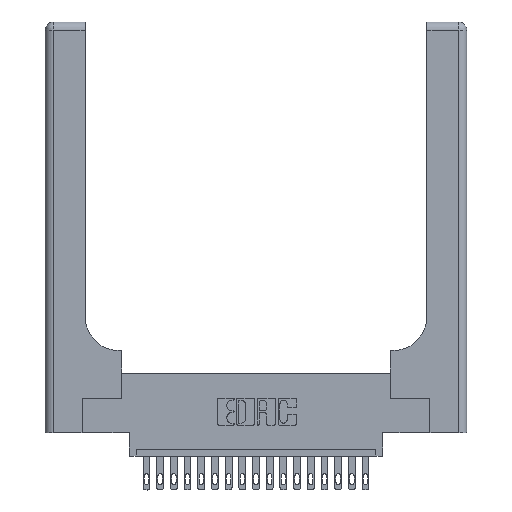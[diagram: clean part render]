
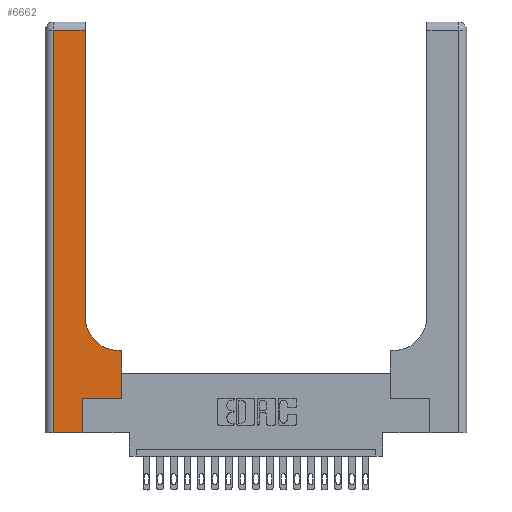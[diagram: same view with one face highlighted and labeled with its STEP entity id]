
A CAD part, top view. The second image highlights one B-rep face of the part: STEP entity #6662.
In plain terms, the highlighted planar face has unit normal (0, 0, 1).
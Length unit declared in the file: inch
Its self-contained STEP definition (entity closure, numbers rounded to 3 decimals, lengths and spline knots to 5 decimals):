
#246 = VERTEX_POINT ( 'NONE', #11468 ) ;
#297 = AXIS2_PLACEMENT_3D ( 'NONE', #9829, #3132, #6411 ) ;
#403 = CARTESIAN_POINT ( 'NONE',  ( 0.06, 2.94, 0.37 ) ) ;
#512 = DIRECTION ( 'NONE',  ( 1., 0., 0. ) ) ;
#562 = EDGE_CURVE ( 'NONE', #246, #17975, #20548, .T. ) ;
#653 = EDGE_CURVE ( 'NONE', #13117, #12980, #16657, .T. ) ;
#734 = LINE ( 'NONE', #16051, #17834 ) ;
#757 = FACE_OUTER_BOUND ( 'NONE', #13804, .T. ) ;
#779 = EDGE_CURVE ( 'NONE', #16602, #246, #13277, .T. ) ;
#911 = ORIENTED_EDGE ( 'NONE', *, *, #779, .T. ) ;
#968 = DIRECTION ( 'NONE',  ( 0., 0., -1. ) ) ;
#2303 = DIRECTION ( 'NONE',  ( -1., 0., 0. ) ) ;
#2444 = CARTESIAN_POINT ( 'NONE',  ( 0.5585, 0.25, 0.37 ) ) ;
#2636 = ORIENTED_EDGE ( 'NONE', *, *, #11655, .T. ) ;
#2727 = CARTESIAN_POINT ( 'NONE',  ( 0.2915, 3., 0.37 ) ) ;
#3095 = CARTESIAN_POINT ( 'NONE',  ( 0.5585, 0.6, 0.37 ) ) ;
#3132 = DIRECTION ( 'NONE',  ( 0., 0., -1. ) ) ;
#3978 = CARTESIAN_POINT ( 'NONE',  ( 0., 2.94, 0.37 ) ) ;
#4124 = DIRECTION ( 'NONE',  ( 0., 1., 0. ) ) ;
#4159 = DIRECTION ( 'NONE',  ( -1., 0., 0. ) ) ;
#4553 = DIRECTION ( 'NONE',  ( 0., 1., 0. ) ) ;
#4919 = CARTESIAN_POINT ( 'NONE',  ( 0.06, 0., 0.37 ) ) ;
#5031 = VECTOR ( 'NONE', #4124, 39.37008 ) ;
#5256 = LINE ( 'NONE', #18958, #9938 ) ;
#5373 = VECTOR ( 'NONE', #15558, 39.37008 ) ;
#6073 = CARTESIAN_POINT ( 'NONE',  ( 0.5415, 0.6, 0.37 ) ) ;
#6411 = DIRECTION ( 'NONE',  ( -1., 0., 0. ) ) ;
#6436 = LINE ( 'NONE', #7379, #10085 ) ;
#6510 = CARTESIAN_POINT ( 'NONE',  ( 0.269, 0., 0.37 ) ) ;
#6606 = CARTESIAN_POINT ( 'NONE',  ( 0.2915, 0.85, 0.37 ) ) ;
#6662 = ADVANCED_FACE ( 'NONE', ( #757 ), #13162, .F. ) ;
#6700 = ORIENTED_EDGE ( 'NONE', *, *, #13232, .T. ) ;
#7112 = VECTOR ( 'NONE', #4553, 39.37008 ) ;
#7288 = EDGE_CURVE ( 'NONE', #17975, #7459, #734, .T. ) ;
#7379 = CARTESIAN_POINT ( 'NONE',  ( 0.2915, 0.6, 0.37 ) ) ;
#7407 = VERTEX_POINT ( 'NONE', #6073 ) ;
#7436 = LINE ( 'NONE', #16893, #14916 ) ;
#7459 = VERTEX_POINT ( 'NONE', #4919 ) ;
#7525 = ORIENTED_EDGE ( 'NONE', *, *, #653, .T. ) ;
#8927 = ORIENTED_EDGE ( 'NONE', *, *, #18132, .T. ) ;
#9523 = DIRECTION ( 'NONE',  ( 0., -1., 0. ) ) ;
#9691 = CARTESIAN_POINT ( 'NONE',  ( 0.269, 0.25, 0.37 ) ) ;
#9829 = CARTESIAN_POINT ( 'NONE',  ( 0., 3., 0.37 ) ) ;
#9938 = VECTOR ( 'NONE', #512, 39.37008 ) ;
#10076 = CARTESIAN_POINT ( 'NONE',  ( 0.5585, 0.25, 0.37 ) ) ;
#10085 = VECTOR ( 'NONE', #4159, 39.37008 ) ;
#10333 = EDGE_CURVE ( 'NONE', #11834, #13117, #5256, .T. ) ;
#11468 = CARTESIAN_POINT ( 'NONE',  ( 0.2915, 2.94, 0.37 ) ) ;
#11655 = EDGE_CURVE ( 'NONE', #7407, #16602, #12904, .T. ) ;
#11767 = VECTOR ( 'NONE', #2303, 39.37008 ) ;
#11834 = VERTEX_POINT ( 'NONE', #9691 ) ;
#12904 = CIRCLE ( 'NONE', #19052, 0.25 ) ;
#12980 = VERTEX_POINT ( 'NONE', #3095 ) ;
#13117 = VERTEX_POINT ( 'NONE', #10076 ) ;
#13119 = DIRECTION ( 'NONE',  ( 1., 0., 0. ) ) ;
#13162 = PLANE ( 'NONE',  #297 ) ;
#13232 = EDGE_CURVE ( 'NONE', #7459, #17883, #7436, .T. ) ;
#13277 = LINE ( 'NONE', #2727, #7112 ) ;
#13321 = ORIENTED_EDGE ( 'NONE', *, *, #7288, .T. ) ;
#13410 = ORIENTED_EDGE ( 'NONE', *, *, #562, .T. ) ;
#13665 = ORIENTED_EDGE ( 'NONE', *, *, #18841, .T. ) ;
#13804 = EDGE_LOOP ( 'NONE', ( #911, #13410, #13321, #6700, #13665, #14671, #7525, #8927, #2636 ) ) ;
#14182 = CARTESIAN_POINT ( 'NONE',  ( 0.269, 0., 0.37 ) ) ;
#14671 = ORIENTED_EDGE ( 'NONE', *, *, #10333, .T. ) ;
#14916 = VECTOR ( 'NONE', #20157, 39.37008 ) ;
#15558 = DIRECTION ( 'NONE',  ( 0., 1., 0. ) ) ;
#16051 = CARTESIAN_POINT ( 'NONE',  ( 0.06, 3., 0.37 ) ) ;
#16154 = CARTESIAN_POINT ( 'NONE',  ( 0.5415, 0.85, 0.37 ) ) ;
#16602 = VERTEX_POINT ( 'NONE', #6606 ) ;
#16657 = LINE ( 'NONE', #2444, #5031 ) ;
#16893 = CARTESIAN_POINT ( 'NONE',  ( 0., 0., 0.37 ) ) ;
#17834 = VECTOR ( 'NONE', #9523, 39.37008 ) ;
#17883 = VERTEX_POINT ( 'NONE', #6510 ) ;
#17975 = VERTEX_POINT ( 'NONE', #403 ) ;
#18132 = EDGE_CURVE ( 'NONE', #12980, #7407, #6436, .T. ) ;
#18841 = EDGE_CURVE ( 'NONE', #17883, #11834, #20358, .T. ) ;
#18958 = CARTESIAN_POINT ( 'NONE',  ( 0.269, 0.25, 0.37 ) ) ;
#19052 = AXIS2_PLACEMENT_3D ( 'NONE', #16154, #968, #13119 ) ;
#20157 = DIRECTION ( 'NONE',  ( 1., 0., 0. ) ) ;
#20358 = LINE ( 'NONE', #14182, #5373 ) ;
#20548 = LINE ( 'NONE', #3978, #11767 ) ;
